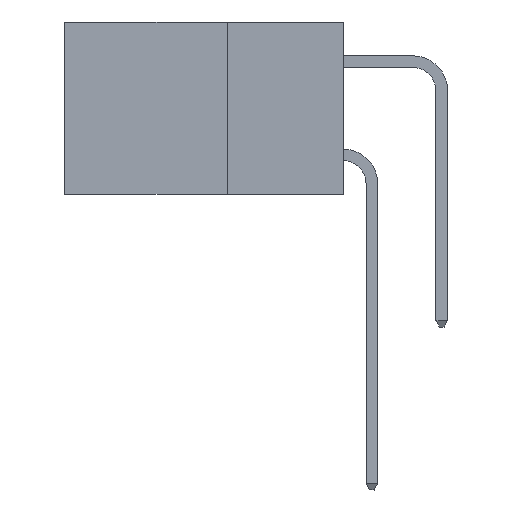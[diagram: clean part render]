
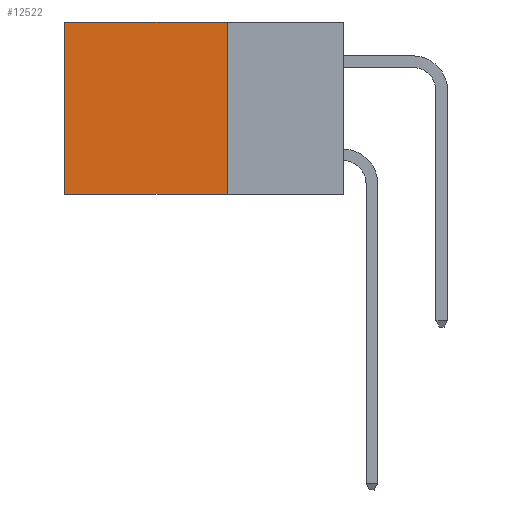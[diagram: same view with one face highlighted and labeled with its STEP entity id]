
A CAD part, left-side view. The second image highlights one B-rep face of the part: STEP entity #12522.
In plain terms, the highlighted planar face has unit normal (-1, 0, 0).
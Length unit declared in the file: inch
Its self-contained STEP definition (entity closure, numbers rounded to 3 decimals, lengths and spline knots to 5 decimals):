
#213 = VERTEX_POINT ( 'NONE', #18784 ) ;
#254 = CARTESIAN_POINT ( 'NONE',  ( 0.298, 0.25, -0.37 ) ) ;
#1868 = VERTEX_POINT ( 'NONE', #2058 ) ;
#2058 = CARTESIAN_POINT ( 'NONE',  ( 0.298, 0.25, 0. ) ) ;
#3132 = CARTESIAN_POINT ( 'NONE',  ( 0.298, 0.6, 0. ) ) ;
#4421 = LINE ( 'NONE', #19031, #15908 ) ;
#4435 = ORIENTED_EDGE ( 'NONE', *, *, #10290, .F. ) ;
#4524 = EDGE_CURVE ( 'NONE', #14106, #213, #12372, .T. ) ;
#6326 = ORIENTED_EDGE ( 'NONE', *, *, #13413, .T. ) ;
#6361 = CARTESIAN_POINT ( 'NONE',  ( 0.298, 0.6, 0. ) ) ;
#7429 = EDGE_CURVE ( 'NONE', #11713, #213, #10295, .T. ) ;
#7432 = ORIENTED_EDGE ( 'NONE', *, *, #7429, .T. ) ;
#8733 = ORIENTED_EDGE ( 'NONE', *, *, #4524, .F. ) ;
#9350 = AXIS2_PLACEMENT_3D ( 'NONE', #12606, #17004, #15584 ) ;
#9664 = DIRECTION ( 'NONE',  ( 0., 0., -1. ) ) ;
#10290 = EDGE_CURVE ( 'NONE', #1868, #14106, #11351, .T. ) ;
#10295 = LINE ( 'NONE', #6361, #17708 ) ;
#11351 = LINE ( 'NONE', #12030, #18765 ) ;
#11511 = FACE_OUTER_BOUND ( 'NONE', #18682, .T. ) ;
#11713 = VERTEX_POINT ( 'NONE', #3132 ) ;
#12030 = CARTESIAN_POINT ( 'NONE',  ( 0.298, 0.25, 0. ) ) ;
#12372 = LINE ( 'NONE', #14060, #15846 ) ;
#12522 = ADVANCED_FACE ( 'NONE', ( #11511 ), #14131, .F. ) ;
#12606 = CARTESIAN_POINT ( 'NONE',  ( 0.298, 0.25, 0. ) ) ;
#13413 = EDGE_CURVE ( 'NONE', #1868, #11713, #4421, .T. ) ;
#13536 = DIRECTION ( 'NONE',  ( 0., 0., -1. ) ) ;
#14060 = CARTESIAN_POINT ( 'NONE',  ( 0.298, 0.25, -0.37 ) ) ;
#14106 = VERTEX_POINT ( 'NONE', #254 ) ;
#14131 = PLANE ( 'NONE',  #9350 ) ;
#14727 = DIRECTION ( 'NONE',  ( 0., 1., 0. ) ) ;
#15584 = DIRECTION ( 'NONE',  ( 0., 0., -1. ) ) ;
#15846 = VECTOR ( 'NONE', #18391, 39.37008 ) ;
#15908 = VECTOR ( 'NONE', #14727, 39.37008 ) ;
#17004 = DIRECTION ( 'NONE',  ( 1., 0., 0. ) ) ;
#17708 = VECTOR ( 'NONE', #9664, 39.37008 ) ;
#18391 = DIRECTION ( 'NONE',  ( 0., 1., 0. ) ) ;
#18682 = EDGE_LOOP ( 'NONE', ( #7432, #8733, #4435, #6326 ) ) ;
#18765 = VECTOR ( 'NONE', #13536, 39.37008 ) ;
#18784 = CARTESIAN_POINT ( 'NONE',  ( 0.298, 0.6, -0.37 ) ) ;
#19031 = CARTESIAN_POINT ( 'NONE',  ( 0.298, 0.25, 0. ) ) ;
